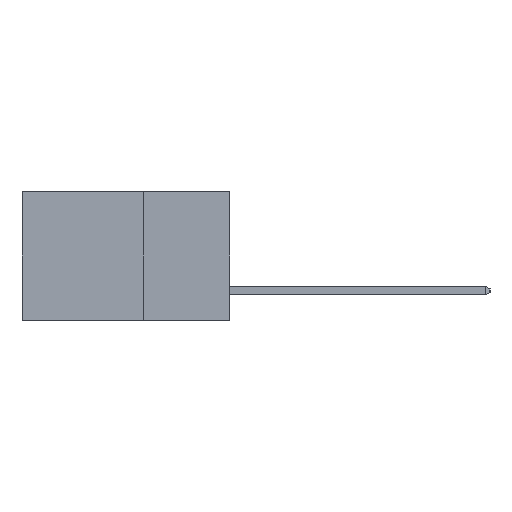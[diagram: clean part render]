
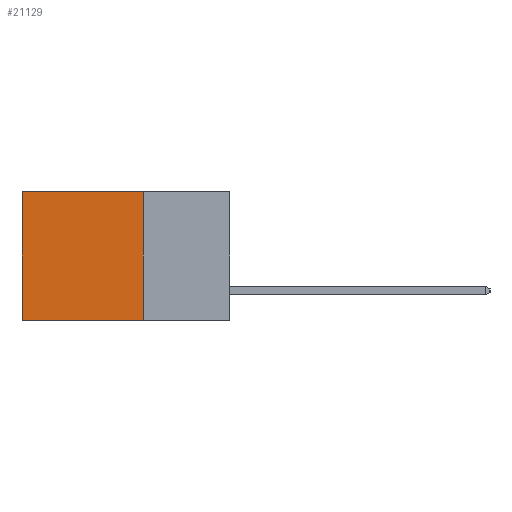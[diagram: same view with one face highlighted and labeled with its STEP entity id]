
A CAD part, left-side view. The second image highlights one B-rep face of the part: STEP entity #21129.
In plain terms, the highlighted planar face has unit normal (-1, 0, 0).
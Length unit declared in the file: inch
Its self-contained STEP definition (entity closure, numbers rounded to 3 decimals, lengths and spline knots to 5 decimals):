
#30 = AXIS2_PLACEMENT_3D ( 'NONE', #20484, #22424, #10826 ) ;
#2125 = FACE_OUTER_BOUND ( 'NONE', #10873, .T. ) ;
#2232 = CARTESIAN_POINT ( 'NONE',  ( 0.298, 0.25, 0. ) ) ;
#2305 = VECTOR ( 'NONE', #18931, 39.37008 ) ;
#2777 = CARTESIAN_POINT ( 'NONE',  ( 0.298, 0.6, 0. ) ) ;
#2930 = CARTESIAN_POINT ( 'NONE',  ( 0.298, 0.6, 0. ) ) ;
#3549 = VERTEX_POINT ( 'NONE', #22663 ) ;
#3983 = EDGE_CURVE ( 'NONE', #3549, #9432, #24881, .T. ) ;
#4128 = ORIENTED_EDGE ( 'NONE', *, *, #21000, .F. ) ;
#4526 = CARTESIAN_POINT ( 'NONE',  ( 0.298, 0.6, -0.37 ) ) ;
#4855 = DIRECTION ( 'NONE',  ( 0., 0., -1. ) ) ;
#4923 = VERTEX_POINT ( 'NONE', #4526 ) ;
#5086 = ORIENTED_EDGE ( 'NONE', *, *, #3983, .F. ) ;
#5201 = LINE ( 'NONE', #22017, #14358 ) ;
#5341 = CARTESIAN_POINT ( 'NONE',  ( 0.298, 0.25, 0. ) ) ;
#5644 = ORIENTED_EDGE ( 'NONE', *, *, #8320, .T. ) ;
#8320 = EDGE_CURVE ( 'NONE', #3549, #14748, #22347, .T. ) ;
#9375 = LINE ( 'NONE', #2777, #23005 ) ;
#9432 = VERTEX_POINT ( 'NONE', #16726 ) ;
#9460 = VECTOR ( 'NONE', #4855, 39.37008 ) ;
#10826 = DIRECTION ( 'NONE',  ( 0., 0., -1. ) ) ;
#10873 = EDGE_LOOP ( 'NONE', ( #13103, #4128, #5086, #5644 ) ) ;
#12571 = DIRECTION ( 'NONE',  ( 0., 0., -1. ) ) ;
#13103 = ORIENTED_EDGE ( 'NONE', *, *, #22768, .T. ) ;
#14358 = VECTOR ( 'NONE', #18267, 39.37008 ) ;
#14748 = VERTEX_POINT ( 'NONE', #2930 ) ;
#16726 = CARTESIAN_POINT ( 'NONE',  ( 0.298, 0.25, -0.37 ) ) ;
#18267 = DIRECTION ( 'NONE',  ( 0., 1., 0. ) ) ;
#18590 = PLANE ( 'NONE',  #30 ) ;
#18931 = DIRECTION ( 'NONE',  ( 0., 1., 0. ) ) ;
#20484 = CARTESIAN_POINT ( 'NONE',  ( 0.298, 0.25, 0. ) ) ;
#21000 = EDGE_CURVE ( 'NONE', #9432, #4923, #5201, .T. ) ;
#21129 = ADVANCED_FACE ( 'NONE', ( #2125 ), #18590, .F. ) ;
#22017 = CARTESIAN_POINT ( 'NONE',  ( 0.298, 0.25, -0.37 ) ) ;
#22347 = LINE ( 'NONE', #5341, #2305 ) ;
#22424 = DIRECTION ( 'NONE',  ( 1., 0., 0. ) ) ;
#22663 = CARTESIAN_POINT ( 'NONE',  ( 0.298, 0.25, 0. ) ) ;
#22768 = EDGE_CURVE ( 'NONE', #14748, #4923, #9375, .T. ) ;
#23005 = VECTOR ( 'NONE', #12571, 39.37008 ) ;
#24881 = LINE ( 'NONE', #2232, #9460 ) ;
